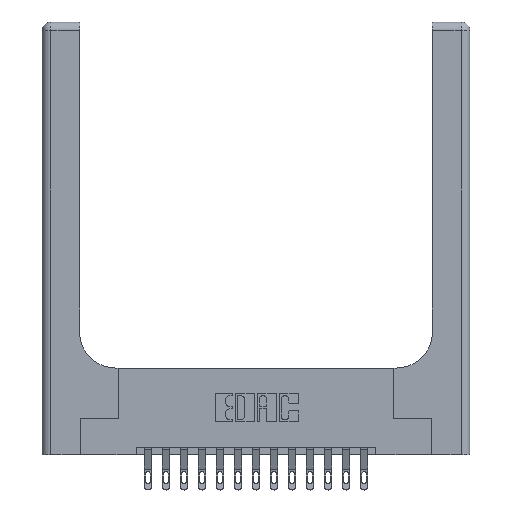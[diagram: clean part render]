
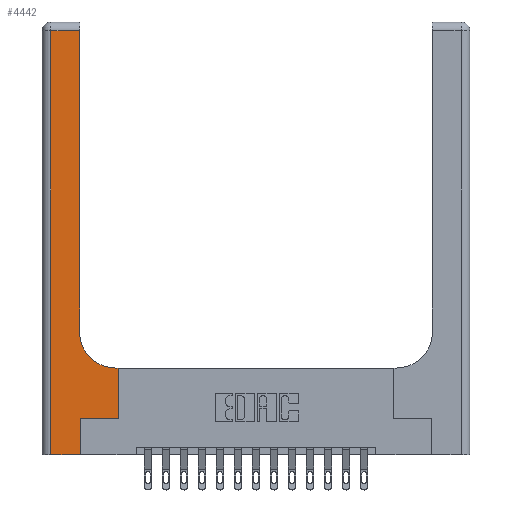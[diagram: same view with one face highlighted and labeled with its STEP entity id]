
A CAD part, top view. The second image highlights one B-rep face of the part: STEP entity #4442.
In plain terms, the highlighted planar face has unit normal (0, 0, 1).
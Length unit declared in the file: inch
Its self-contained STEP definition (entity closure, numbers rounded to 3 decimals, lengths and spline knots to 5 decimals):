
#1091 = AXIS2_PLACEMENT_3D ( 'NONE', #13434, #17415, #16012 ) ;
#1217 = EDGE_CURVE ( 'NONE', #8545, #9704, #12475, .T. ) ;
#1234 = EDGE_CURVE ( 'NONE', #14580, #11753, #18102, .T. ) ;
#1245 = LINE ( 'NONE', #18218, #1715 ) ;
#1280 = ORIENTED_EDGE ( 'NONE', *, *, #1489, .T. ) ;
#1489 = EDGE_CURVE ( 'NONE', #3970, #2566, #12119, .T. ) ;
#1715 = VECTOR ( 'NONE', #5499, 39.37008 ) ;
#2344 = VERTEX_POINT ( 'NONE', #7287 ) ;
#2360 = CARTESIAN_POINT ( 'NONE',  ( 0., 2.94, 0.37 ) ) ;
#2508 = ORIENTED_EDGE ( 'NONE', *, *, #1234, .T. ) ;
#2566 = VERTEX_POINT ( 'NONE', #13744 ) ;
#2635 = VECTOR ( 'NONE', #12075, 39.37008 ) ;
#3453 = ORIENTED_EDGE ( 'NONE', *, *, #15642, .T. ) ;
#3684 = CARTESIAN_POINT ( 'NONE',  ( 0.26, 3., 0.37 ) ) ;
#3866 = VECTOR ( 'NONE', #16599, 39.37008 ) ;
#3970 = VERTEX_POINT ( 'NONE', #10742 ) ;
#4153 = ORIENTED_EDGE ( 'NONE', *, *, #5245, .T. ) ;
#4389 = ORIENTED_EDGE ( 'NONE', *, *, #8894, .T. ) ;
#4442 = ADVANCED_FACE ( 'NONE', ( #6107 ), #16296, .F. ) ;
#4526 = ORIENTED_EDGE ( 'NONE', *, *, #17554, .T. ) ;
#4909 = LINE ( 'NONE', #13726, #2635 ) ;
#4979 = EDGE_CURVE ( 'NONE', #2344, #8545, #1245, .T. ) ;
#5114 = ORIENTED_EDGE ( 'NONE', *, *, #16647, .T. ) ;
#5212 = CARTESIAN_POINT ( 'NONE',  ( 0.51, 0.6, 0.37 ) ) ;
#5245 = EDGE_CURVE ( 'NONE', #8455, #2344, #14006, .T. ) ;
#5499 = DIRECTION ( 'NONE',  ( -1., 0., 0. ) ) ;
#6107 = FACE_OUTER_BOUND ( 'NONE', #14541, .T. ) ;
#6547 = DIRECTION ( 'NONE',  ( 0., 1., 0. ) ) ;
#7287 = CARTESIAN_POINT ( 'NONE',  ( 0.528, 0.6, 0.37 ) ) ;
#7655 = LINE ( 'NONE', #15781, #16813 ) ;
#7660 = DIRECTION ( 'NONE',  ( 0., 0., -1. ) ) ;
#7860 = CARTESIAN_POINT ( 'NONE',  ( 0.51, 0.85, 0.37 ) ) ;
#8410 = CARTESIAN_POINT ( 'NONE',  ( 0.06, 3., 0.37 ) ) ;
#8455 = VERTEX_POINT ( 'NONE', #9004 ) ;
#8484 = CARTESIAN_POINT ( 'NONE',  ( 0.528, 0.25, 0.37 ) ) ;
#8545 = VERTEX_POINT ( 'NONE', #5212 ) ;
#8749 = CARTESIAN_POINT ( 'NONE',  ( 0.26, 0.85, 0.37 ) ) ;
#8894 = EDGE_CURVE ( 'NONE', #11753, #3970, #7655, .T. ) ;
#9004 = CARTESIAN_POINT ( 'NONE',  ( 0.528, 0.25, 0.37 ) ) ;
#9552 = VECTOR ( 'NONE', #9663, 39.37008 ) ;
#9663 = DIRECTION ( 'NONE',  ( -1., 0., 0. ) ) ;
#9704 = VERTEX_POINT ( 'NONE', #8749 ) ;
#9997 = ORIENTED_EDGE ( 'NONE', *, *, #1217, .T. ) ;
#10293 = DIRECTION ( 'NONE',  ( 1., 0., 0. ) ) ;
#10742 = CARTESIAN_POINT ( 'NONE',  ( 0.265, 0., 0.37 ) ) ;
#10780 = CARTESIAN_POINT ( 'NONE',  ( 0.265, 0., 0.37 ) ) ;
#10806 = CARTESIAN_POINT ( 'NONE',  ( 0.06, 2.94, 0.37 ) ) ;
#11330 = AXIS2_PLACEMENT_3D ( 'NONE', #7860, #7660, #11922 ) ;
#11556 = VECTOR ( 'NONE', #14086, 39.37008 ) ;
#11712 = CARTESIAN_POINT ( 'NONE',  ( 0.26, 2.94, 0.37 ) ) ;
#11753 = VERTEX_POINT ( 'NONE', #12954 ) ;
#11922 = DIRECTION ( 'NONE',  ( 1., 0., 0. ) ) ;
#12075 = DIRECTION ( 'NONE',  ( 1., 0., 0. ) ) ;
#12119 = LINE ( 'NONE', #10780, #16015 ) ;
#12370 = ORIENTED_EDGE ( 'NONE', *, *, #4979, .T. ) ;
#12475 = CIRCLE ( 'NONE', #11330, 0.25 ) ;
#12954 = CARTESIAN_POINT ( 'NONE',  ( 0.06, 0., 0.37 ) ) ;
#13434 = CARTESIAN_POINT ( 'NONE',  ( 0., 3., 0.37 ) ) ;
#13726 = CARTESIAN_POINT ( 'NONE',  ( 0.265, 0.25, 0.37 ) ) ;
#13744 = CARTESIAN_POINT ( 'NONE',  ( 0.265, 0.25, 0.37 ) ) ;
#14006 = LINE ( 'NONE', #8484, #11556 ) ;
#14086 = DIRECTION ( 'NONE',  ( 0., 1., 0. ) ) ;
#14541 = EDGE_LOOP ( 'NONE', ( #3453, #4526, #2508, #4389, #1280, #5114, #4153, #12370, #9997 ) ) ;
#14580 = VERTEX_POINT ( 'NONE', #10806 ) ;
#14747 = VECTOR ( 'NONE', #17713, 39.37008 ) ;
#15642 = EDGE_CURVE ( 'NONE', #9704, #16881, #17807, .T. ) ;
#15781 = CARTESIAN_POINT ( 'NONE',  ( 0., 0., 0.37 ) ) ;
#16012 = DIRECTION ( 'NONE',  ( -1., 0., 0. ) ) ;
#16015 = VECTOR ( 'NONE', #6547, 39.37008 ) ;
#16296 = PLANE ( 'NONE',  #1091 ) ;
#16599 = DIRECTION ( 'NONE',  ( 0., -1., 0. ) ) ;
#16647 = EDGE_CURVE ( 'NONE', #2566, #8455, #4909, .T. ) ;
#16813 = VECTOR ( 'NONE', #10293, 39.37008 ) ;
#16881 = VERTEX_POINT ( 'NONE', #11712 ) ;
#17415 = DIRECTION ( 'NONE',  ( 0., 0., -1. ) ) ;
#17554 = EDGE_CURVE ( 'NONE', #16881, #14580, #18126, .T. ) ;
#17713 = DIRECTION ( 'NONE',  ( 0., 1., 0. ) ) ;
#17807 = LINE ( 'NONE', #3684, #14747 ) ;
#18102 = LINE ( 'NONE', #8410, #3866 ) ;
#18126 = LINE ( 'NONE', #2360, #9552 ) ;
#18218 = CARTESIAN_POINT ( 'NONE',  ( 0.26, 0.6, 0.37 ) ) ;
